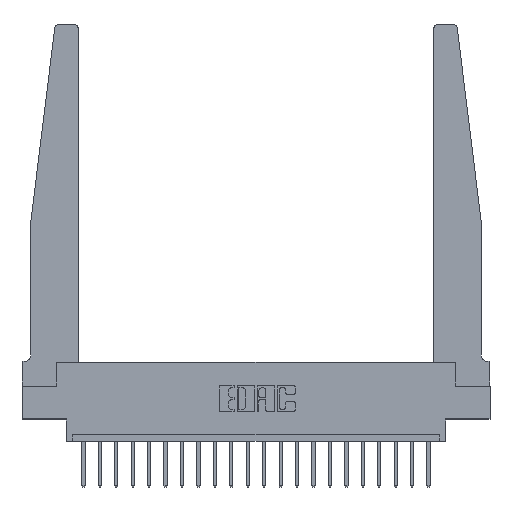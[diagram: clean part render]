
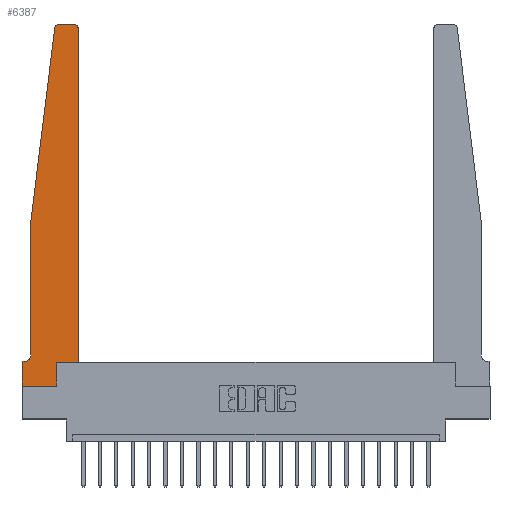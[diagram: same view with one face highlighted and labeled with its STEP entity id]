
A CAD part, top view. The second image highlights one B-rep face of the part: STEP entity #6387.
In plain terms, the highlighted planar face has unit normal (0, 0, 1).
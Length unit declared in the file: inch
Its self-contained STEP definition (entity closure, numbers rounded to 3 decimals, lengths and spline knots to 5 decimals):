
#222 = EDGE_CURVE ( 'NONE', #504, #2126, #15925, .T. ) ;
#304 = AXIS2_PLACEMENT_3D ( 'NONE', #16253, #17857, #19632 ) ;
#338 = CARTESIAN_POINT ( 'NONE',  ( 0.425, 2.72, 0.37 ) ) ;
#504 = VERTEX_POINT ( 'NONE', #20020 ) ;
#696 = LINE ( 'NONE', #2622, #17631 ) ;
#834 = EDGE_LOOP ( 'NONE', ( #18855, #8553, #14774, #5744, #5230, #1300, #12065, #3808, #839, #8078, #10354, #5718 ) ) ;
#839 = ORIENTED_EDGE ( 'NONE', *, *, #10078, .T. ) ;
#924 = CARTESIAN_POINT ( 'NONE',  ( 0.27653, 2.72, 0.37 ) ) ;
#1300 = ORIENTED_EDGE ( 'NONE', *, *, #18592, .T. ) ;
#2126 = VERTEX_POINT ( 'NONE', #5062 ) ;
#2622 = CARTESIAN_POINT ( 'NONE',  ( 0., 0., 0.37 ) ) ;
#2630 = DIRECTION ( 'NONE',  ( 1., 0., 0. ) ) ;
#3097 = CARTESIAN_POINT ( 'NONE',  ( 0.395, 2.75, 0.37 ) ) ;
#3558 = LINE ( 'NONE', #12777, #13786 ) ;
#3625 = CARTESIAN_POINT ( 'NONE',  ( 0.25, 2.75, 0.37 ) ) ;
#3712 = VECTOR ( 'NONE', #9509, 39.37008 ) ;
#3782 = DIRECTION ( 'NONE',  ( -1., 0., 0. ) ) ;
#3808 = ORIENTED_EDGE ( 'NONE', *, *, #20609, .T. ) ;
#3826 = CARTESIAN_POINT ( 'NONE',  ( 0.425, 0.18, 0.37 ) ) ;
#3842 = DIRECTION ( 'NONE',  ( 1., 0., 0. ) ) ;
#3991 = CARTESIAN_POINT ( 'NONE',  ( 0.395, 2.72, 0.37 ) ) ;
#4510 = LINE ( 'NONE', #15150, #16835 ) ;
#4530 = LINE ( 'NONE', #5646, #7163 ) ;
#5062 = CARTESIAN_POINT ( 'NONE',  ( 0.015, 0.1875, 0.37 ) ) ;
#5096 = VECTOR ( 'NONE', #15513, 39.37008 ) ;
#5230 = ORIENTED_EDGE ( 'NONE', *, *, #222, .T. ) ;
#5646 = CARTESIAN_POINT ( 'NONE',  ( 0.065, 0.1875, 0.37 ) ) ;
#5718 = ORIENTED_EDGE ( 'NONE', *, *, #20466, .T. ) ;
#5744 = ORIENTED_EDGE ( 'NONE', *, *, #20892, .T. ) ;
#6387 = ADVANCED_FACE ( 'NONE', ( #17630 ), #19566, .T. ) ;
#6913 = VERTEX_POINT ( 'NONE', #9374 ) ;
#6934 = CARTESIAN_POINT ( 'NONE',  ( 0., 0., 0.37 ) ) ;
#7163 = VECTOR ( 'NONE', #20343, 39.37008 ) ;
#7373 = DIRECTION ( 'NONE',  ( 0., -1., 0. ) ) ;
#7520 = EDGE_CURVE ( 'NONE', #13722, #11697, #3558, .T. ) ;
#7971 = CARTESIAN_POINT ( 'NONE',  ( 0.425, 0.18, 0.37 ) ) ;
#8078 = ORIENTED_EDGE ( 'NONE', *, *, #15475, .T. ) ;
#8133 = EDGE_CURVE ( 'NONE', #8631, #15883, #8181, .T. ) ;
#8164 = AXIS2_PLACEMENT_3D ( 'NONE', #19257, #18967, #15738 ) ;
#8181 = LINE ( 'NONE', #9856, #5096 ) ;
#8354 = CIRCLE ( 'NONE', #12832, 0.03 ) ;
#8498 = DIRECTION ( 'NONE',  ( 0., 1., 0. ) ) ;
#8553 = ORIENTED_EDGE ( 'NONE', *, *, #11412, .T. ) ;
#8631 = VERTEX_POINT ( 'NONE', #11791 ) ;
#9374 = CARTESIAN_POINT ( 'NONE',  ( 0.2605, 0., 0.37 ) ) ;
#9509 = DIRECTION ( 'NONE',  ( 1., 0., 0. ) ) ;
#9856 = CARTESIAN_POINT ( 'NONE',  ( 0.065, 1.25, 0.37 ) ) ;
#10061 = CARTESIAN_POINT ( 'NONE',  ( 0.2605, 0.18, 0.37 ) ) ;
#10078 = EDGE_CURVE ( 'NONE', #6913, #18022, #4510, .T. ) ;
#10268 = EDGE_CURVE ( 'NONE', #18231, #18513, #14072, .T. ) ;
#10354 = ORIENTED_EDGE ( 'NONE', *, *, #7520, .T. ) ;
#10687 = DIRECTION ( 'NONE',  ( 1., 0., 0. ) ) ;
#11220 = VECTOR ( 'NONE', #7373, 39.37008 ) ;
#11412 = EDGE_CURVE ( 'NONE', #14088, #8631, #17328, .T. ) ;
#11697 = VERTEX_POINT ( 'NONE', #338 ) ;
#11757 = DIRECTION ( 'NONE',  ( 0., 1., 0. ) ) ;
#11791 = CARTESIAN_POINT ( 'NONE',  ( 0.24675, 2.72367, 0.37 ) ) ;
#12065 = ORIENTED_EDGE ( 'NONE', *, *, #10268, .T. ) ;
#12777 = CARTESIAN_POINT ( 'NONE',  ( 0.425, 0.18, 0.37 ) ) ;
#12832 = AXIS2_PLACEMENT_3D ( 'NONE', #3991, #20124, #3842 ) ;
#13686 = VECTOR ( 'NONE', #19599, 39.37008 ) ;
#13722 = VERTEX_POINT ( 'NONE', #3826 ) ;
#13786 = VECTOR ( 'NONE', #8498, 39.37008 ) ;
#13984 = CARTESIAN_POINT ( 'NONE',  ( 0., 0., 0.37 ) ) ;
#14072 = LINE ( 'NONE', #13984, #11220 ) ;
#14088 = VERTEX_POINT ( 'NONE', #19622 ) ;
#14209 = LINE ( 'NONE', #19750, #13686 ) ;
#14774 = ORIENTED_EDGE ( 'NONE', *, *, #8133, .T. ) ;
#15150 = CARTESIAN_POINT ( 'NONE',  ( 0.2605, 0.18, 0.37 ) ) ;
#15467 = AXIS2_PLACEMENT_3D ( 'NONE', #924, #17290, #2630 ) ;
#15475 = EDGE_CURVE ( 'NONE', #18022, #13722, #18619, .T. ) ;
#15513 = DIRECTION ( 'NONE',  ( -0.122, -0.992, 0. ) ) ;
#15729 = LINE ( 'NONE', #3625, #20790 ) ;
#15738 = DIRECTION ( 'NONE',  ( -1., 0., 0. ) ) ;
#15883 = VERTEX_POINT ( 'NONE', #19638 ) ;
#15925 = CIRCLE ( 'NONE', #8164, 0.05 ) ;
#16253 = CARTESIAN_POINT ( 'NONE',  ( 0., 0.1875, 0.37 ) ) ;
#16835 = VECTOR ( 'NONE', #11757, 39.37008 ) ;
#17290 = DIRECTION ( 'NONE',  ( 0., 0., 1. ) ) ;
#17328 = CIRCLE ( 'NONE', #15467, 0.03 ) ;
#17570 = CARTESIAN_POINT ( 'NONE',  ( 0., 0.1875, 0.37 ) ) ;
#17630 = FACE_OUTER_BOUND ( 'NONE', #834, .T. ) ;
#17631 = VECTOR ( 'NONE', #10687, 39.37008 ) ;
#17857 = DIRECTION ( 'NONE',  ( 0., 0., 1. ) ) ;
#18022 = VERTEX_POINT ( 'NONE', #10061 ) ;
#18231 = VERTEX_POINT ( 'NONE', #17570 ) ;
#18513 = VERTEX_POINT ( 'NONE', #6934 ) ;
#18544 = EDGE_CURVE ( 'NONE', #20718, #14088, #15729, .T. ) ;
#18592 = EDGE_CURVE ( 'NONE', #2126, #18231, #4530, .T. ) ;
#18619 = LINE ( 'NONE', #7971, #3712 ) ;
#18855 = ORIENTED_EDGE ( 'NONE', *, *, #18544, .T. ) ;
#18967 = DIRECTION ( 'NONE',  ( 0., 0., -1. ) ) ;
#19257 = CARTESIAN_POINT ( 'NONE',  ( 0.015, 0.2375, 0.37 ) ) ;
#19566 = PLANE ( 'NONE',  #304 ) ;
#19599 = DIRECTION ( 'NONE',  ( 0., -1., 0. ) ) ;
#19622 = CARTESIAN_POINT ( 'NONE',  ( 0.27653, 2.75, 0.37 ) ) ;
#19632 = DIRECTION ( 'NONE',  ( 1., 0., 0. ) ) ;
#19638 = CARTESIAN_POINT ( 'NONE',  ( 0.065, 1.25, 0.37 ) ) ;
#19750 = CARTESIAN_POINT ( 'NONE',  ( 0.065, 1.25, 0.37 ) ) ;
#20020 = CARTESIAN_POINT ( 'NONE',  ( 0.065, 0.2375, 0.37 ) ) ;
#20124 = DIRECTION ( 'NONE',  ( 0., 0., 1. ) ) ;
#20343 = DIRECTION ( 'NONE',  ( -1., 0., 0. ) ) ;
#20466 = EDGE_CURVE ( 'NONE', #11697, #20718, #8354, .T. ) ;
#20609 = EDGE_CURVE ( 'NONE', #18513, #6913, #696, .T. ) ;
#20718 = VERTEX_POINT ( 'NONE', #3097 ) ;
#20790 = VECTOR ( 'NONE', #3782, 39.37008 ) ;
#20892 = EDGE_CURVE ( 'NONE', #15883, #504, #14209, .T. ) ;
